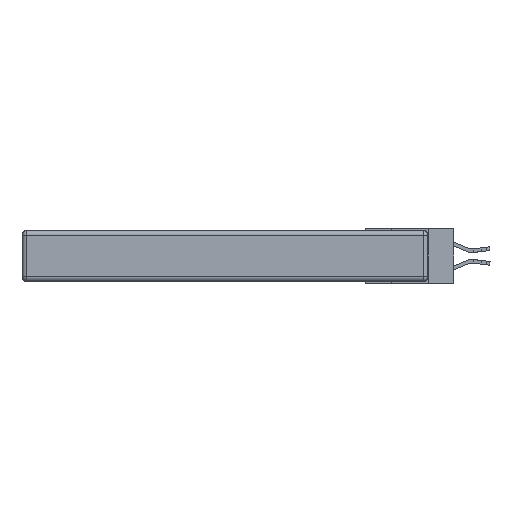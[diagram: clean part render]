
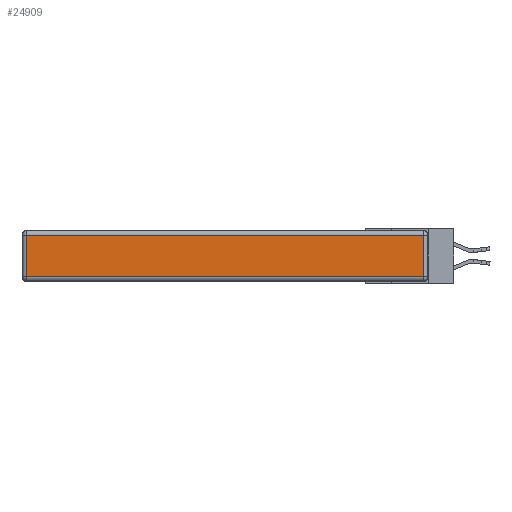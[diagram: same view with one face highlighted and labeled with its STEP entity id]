
A CAD part, left-side view. The second image highlights one B-rep face of the part: STEP entity #24909.
In plain terms, the highlighted planar face has unit normal (-1, 0, 0).
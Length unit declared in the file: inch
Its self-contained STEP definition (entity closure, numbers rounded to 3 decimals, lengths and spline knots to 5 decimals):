
#1627 = PLANE ( 'NONE',  #9736 ) ;
#2656 = VECTOR ( 'NONE', #15314, 39.37008 ) ;
#3144 = DIRECTION ( 'NONE',  ( 0., 0., 1. ) ) ;
#4392 = VECTOR ( 'NONE', #17685, 39.37008 ) ;
#4565 = CARTESIAN_POINT ( 'NONE',  ( 0., 0.03, -0.03 ) ) ;
#5026 = VECTOR ( 'NONE', #3144, 39.37008 ) ;
#6211 = EDGE_CURVE ( 'NONE', #20150, #8003, #21803, .T. ) ;
#7458 = CARTESIAN_POINT ( 'NONE',  ( 0., 0.03, -0.313 ) ) ;
#8003 = VERTEX_POINT ( 'NONE', #26464 ) ;
#8200 = CARTESIAN_POINT ( 'NONE',  ( 0., 0., -0.343 ) ) ;
#9397 = ORIENTED_EDGE ( 'NONE', *, *, #15668, .T. ) ;
#9736 = AXIS2_PLACEMENT_3D ( 'NONE', #8200, #16427, #20500 ) ;
#11972 = LINE ( 'NONE', #17650, #2656 ) ;
#15314 = DIRECTION ( 'NONE',  ( 0., 0., -1. ) ) ;
#15668 = EDGE_CURVE ( 'NONE', #19137, #23376, #26038, .T. ) ;
#16427 = DIRECTION ( 'NONE',  ( -1., 0., 0. ) ) ;
#16987 = CARTESIAN_POINT ( 'NONE',  ( 0., 2.72, -0.313 ) ) ;
#17495 = ORIENTED_EDGE ( 'NONE', *, *, #25502, .T. ) ;
#17650 = CARTESIAN_POINT ( 'NONE',  ( 0., 2.72, -0.343 ) ) ;
#17685 = DIRECTION ( 'NONE',  ( 0., 1., 0. ) ) ;
#18193 = EDGE_CURVE ( 'NONE', #8003, #19137, #11972, .T. ) ;
#18368 = CARTESIAN_POINT ( 'NONE',  ( 0., 0., -0.313 ) ) ;
#18972 = ORIENTED_EDGE ( 'NONE', *, *, #18193, .T. ) ;
#19137 = VERTEX_POINT ( 'NONE', #16987 ) ;
#20150 = VERTEX_POINT ( 'NONE', #4565 ) ;
#20375 = ORIENTED_EDGE ( 'NONE', *, *, #6211, .T. ) ;
#20461 = DIRECTION ( 'NONE',  ( 0., -1., 0. ) ) ;
#20500 = DIRECTION ( 'NONE',  ( 0., 0., 1. ) ) ;
#21781 = LINE ( 'NONE', #21890, #5026 ) ;
#21803 = LINE ( 'NONE', #24200, #4392 ) ;
#21836 = VECTOR ( 'NONE', #20461, 39.37008 ) ;
#21890 = CARTESIAN_POINT ( 'NONE',  ( 0., 0.03, -0.343 ) ) ;
#22111 = EDGE_LOOP ( 'NONE', ( #9397, #17495, #20375, #18972 ) ) ;
#23376 = VERTEX_POINT ( 'NONE', #7458 ) ;
#24200 = CARTESIAN_POINT ( 'NONE',  ( 0., 2.75, -0.03 ) ) ;
#24909 = ADVANCED_FACE ( 'NONE', ( #25393 ), #1627, .T. ) ;
#25393 = FACE_OUTER_BOUND ( 'NONE', #22111, .T. ) ;
#25502 = EDGE_CURVE ( 'NONE', #23376, #20150, #21781, .T. ) ;
#26038 = LINE ( 'NONE', #18368, #21836 ) ;
#26464 = CARTESIAN_POINT ( 'NONE',  ( 0., 2.72, -0.03 ) ) ;
